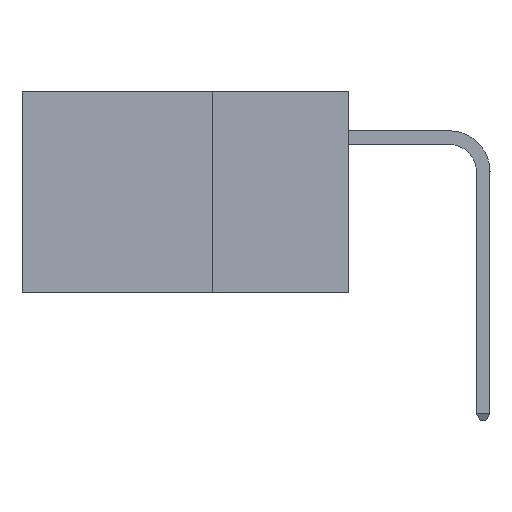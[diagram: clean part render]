
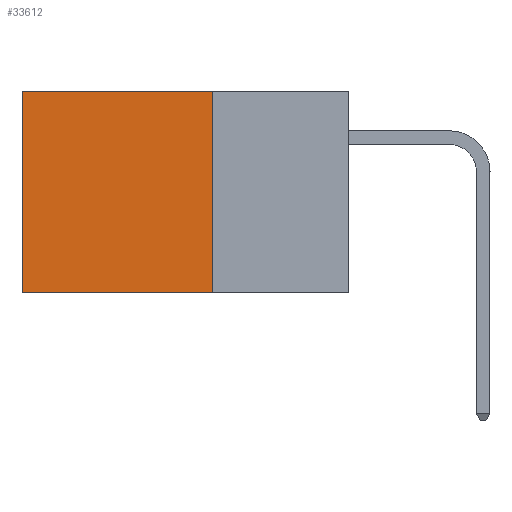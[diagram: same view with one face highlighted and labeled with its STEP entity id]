
A CAD part, left-side view. The second image highlights one B-rep face of the part: STEP entity #33612.
In plain terms, the highlighted planar face has unit normal (-1, 0, 0).
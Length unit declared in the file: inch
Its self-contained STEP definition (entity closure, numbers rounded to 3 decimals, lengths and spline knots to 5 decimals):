
#879 = DIRECTION ( 'NONE',  ( 0., 1., 0. ) ) ;
#1121 = EDGE_CURVE ( 'NONE', #17138, #1605, #37068, .T. ) ;
#1605 = VERTEX_POINT ( 'NONE', #40976 ) ;
#1752 = AXIS2_PLACEMENT_3D ( 'NONE', #24377, #38380, #17485 ) ;
#5289 = VERTEX_POINT ( 'NONE', #8045 ) ;
#5624 = FACE_OUTER_BOUND ( 'NONE', #39210, .T. ) ;
#6950 = VECTOR ( 'NONE', #14753, 39.37008 ) ;
#8045 = CARTESIAN_POINT ( 'NONE',  ( 0.2875, 0.25, -0.37 ) ) ;
#10068 = CARTESIAN_POINT ( 'NONE',  ( 0.2875, 0.6, -0.37 ) ) ;
#12957 = EDGE_CURVE ( 'NONE', #1605, #28514, #32642, .T. ) ;
#14216 = VECTOR ( 'NONE', #25450, 39.37008 ) ;
#14227 = ORIENTED_EDGE ( 'NONE', *, *, #1121, .T. ) ;
#14753 = DIRECTION ( 'NONE',  ( 0., 1., 0. ) ) ;
#16357 = ORIENTED_EDGE ( 'NONE', *, *, #12957, .T. ) ;
#17138 = VERTEX_POINT ( 'NONE', #37421 ) ;
#17485 = DIRECTION ( 'NONE',  ( 0., 0., -1. ) ) ;
#18787 = CARTESIAN_POINT ( 'NONE',  ( 0.2875, 0.25, 0. ) ) ;
#20342 = PLANE ( 'NONE',  #1752 ) ;
#21567 = EDGE_CURVE ( 'NONE', #17138, #5289, #35901, .T. ) ;
#21732 = DIRECTION ( 'NONE',  ( 0., 0., -1. ) ) ;
#24377 = CARTESIAN_POINT ( 'NONE',  ( 0.2875, 0.25, 0. ) ) ;
#25450 = DIRECTION ( 'NONE',  ( 0., 0., -1. ) ) ;
#28514 = VERTEX_POINT ( 'NONE', #10068 ) ;
#32642 = LINE ( 'NONE', #46435, #44049 ) ;
#33612 = ADVANCED_FACE ( 'NONE', ( #5624 ), #20342, .F. ) ;
#34216 = ORIENTED_EDGE ( 'NONE', *, *, #21567, .F. ) ;
#34711 = ORIENTED_EDGE ( 'NONE', *, *, #41818, .F. ) ;
#35901 = LINE ( 'NONE', #43249, #14216 ) ;
#36038 = CARTESIAN_POINT ( 'NONE',  ( 0.2875, 0.25, -0.37 ) ) ;
#36959 = VECTOR ( 'NONE', #879, 39.37008 ) ;
#37068 = LINE ( 'NONE', #18787, #6950 ) ;
#37421 = CARTESIAN_POINT ( 'NONE',  ( 0.2875, 0.25, 0. ) ) ;
#38380 = DIRECTION ( 'NONE',  ( 1., 0., 0. ) ) ;
#39210 = EDGE_LOOP ( 'NONE', ( #16357, #34711, #34216, #14227 ) ) ;
#40057 = LINE ( 'NONE', #36038, #36959 ) ;
#40976 = CARTESIAN_POINT ( 'NONE',  ( 0.2875, 0.6, 0. ) ) ;
#41818 = EDGE_CURVE ( 'NONE', #5289, #28514, #40057, .T. ) ;
#43249 = CARTESIAN_POINT ( 'NONE',  ( 0.2875, 0.25, 0. ) ) ;
#44049 = VECTOR ( 'NONE', #21732, 39.37008 ) ;
#46435 = CARTESIAN_POINT ( 'NONE',  ( 0.2875, 0.6, 0. ) ) ;
